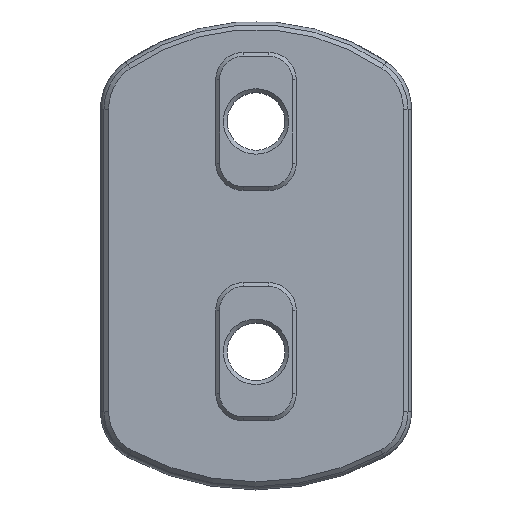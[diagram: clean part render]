
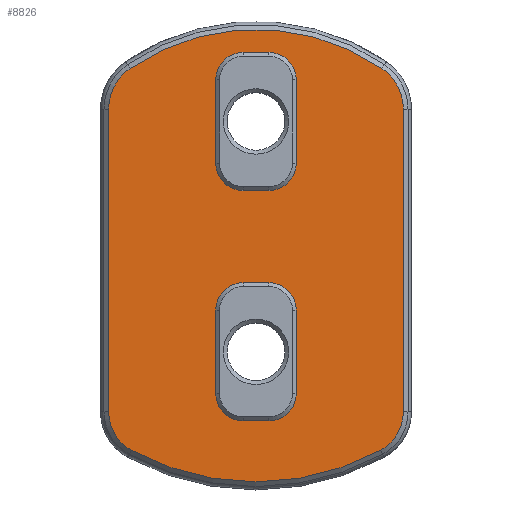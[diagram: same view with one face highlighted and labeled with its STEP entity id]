
A CAD part, top view. The second image highlights one B-rep face of the part: STEP entity #8826.
In plain terms, the highlighted planar face has unit normal (0, 0, 1).
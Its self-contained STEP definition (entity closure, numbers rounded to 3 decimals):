
#85=FACE_BOUND('',#2381,.T.);
#86=FACE_BOUND('',#2382,.T.);
#134=PLANE('',#9695);
#447=LINE('',#20648,#837);
#455=LINE('',#20966,#845);
#470=LINE('',#21016,#860);
#550=LINE('',#22989,#940);
#552=LINE('',#22998,#942);
#553=LINE('',#23002,#943);
#554=LINE('',#23005,#944);
#555=LINE('',#23007,#945);
#556=LINE('',#23009,#946);
#557=LINE('',#23013,#947);
#837=VECTOR('',#11187,10.);
#845=VECTOR('',#11223,10.);
#860=VECTOR('',#11274,10.);
#940=VECTOR('',#11726,10.);
#942=VECTOR('',#11738,10.);
#943=VECTOR('',#11741,10.);
#944=VECTOR('',#11744,10.);
#945=VECTOR('',#11745,10.);
#946=VECTOR('',#11746,10.);
#947=VECTOR('',#11749,10.);
#1774=FACE_OUTER_BOUND('',#2380,.T.);
#2380=EDGE_LOOP('',(#7814,#7815,#7816,#7817,#7818,#7819,#7820,#7821));
#2381=EDGE_LOOP('',(#7822,#7823,#7824,#7825,#7826,#7827,#7828,#7829));
#2382=EDGE_LOOP('',(#7830,#7831,#7832,#7833,#7834,#7835,#7836,#7837));
#2712=B_SPLINE_CURVE_WITH_KNOTS('',3,(#20640,#20641,#20642,#20643,#20644),
 .UNSPECIFIED.,.F.,.F.,(4,1,4),(0.,0.207,0.484),
 .UNSPECIFIED.);
#2804=B_SPLINE_CURVE_WITH_KNOTS('',3,(#22981,#22982,#22983,#22984,#22985),
 .UNSPECIFIED.,.F.,.F.,(4,1,4),(0.,0.207,0.484),
 .UNSPECIFIED.);
#3143=CIRCLE('',#9474,4.3);
#3150=CIRCLE('',#9484,2.38);
#3153=CIRCLE('',#9489,2.38);
#3160=CIRCLE('',#9503,2.38);
#3161=CIRCLE('',#9506,2.38);
#3261=CIRCLE('',#9689,22.602);
#3262=CIRCLE('',#9692,4.3);
#3263=CIRCLE('',#9694,19.302);
#3264=CIRCLE('',#9696,2.38);
#3265=CIRCLE('',#9697,2.38);
#3266=CIRCLE('',#9698,2.38);
#3267=CIRCLE('',#9699,2.38);
#3817=VERTEX_POINT('',#20637);
#3818=VERTEX_POINT('',#20639);
#3819=VERTEX_POINT('',#20647);
#3820=VERTEX_POINT('',#20651);
#3828=VERTEX_POINT('',#20953);
#3829=VERTEX_POINT('',#20954);
#3833=VERTEX_POINT('',#20964);
#3835=VERTEX_POINT('',#20970);
#3848=VERTEX_POINT('',#21009);
#3849=VERTEX_POINT('',#21011);
#3850=VERTEX_POINT('',#21015);
#3851=VERTEX_POINT('',#21019);
#3982=VERTEX_POINT('',#22956);
#3983=VERTEX_POINT('',#22979);
#3984=VERTEX_POINT('',#22987);
#3985=VERTEX_POINT('',#22991);
#3986=VERTEX_POINT('',#22997);
#3987=VERTEX_POINT('',#22999);
#3988=VERTEX_POINT('',#23001);
#3989=VERTEX_POINT('',#23003);
#3990=VERTEX_POINT('',#23006);
#3991=VERTEX_POINT('',#23008);
#3992=VERTEX_POINT('',#23010);
#3993=VERTEX_POINT('',#23012);
#4957=EDGE_CURVE('',#3818,#3817,#2712,.T.);
#4959=EDGE_CURVE('',#3819,#3818,#447,.T.);
#4961=EDGE_CURVE('',#3820,#3819,#3143,.T.);
#4981=EDGE_CURVE('',#3828,#3829,#3150,.T.);
#4987=EDGE_CURVE('',#3829,#3833,#455,.T.);
#4990=EDGE_CURVE('',#3835,#3833,#3153,.T.);
#5009=EDGE_CURVE('',#3849,#3848,#3160,.T.);
#5011=EDGE_CURVE('',#3850,#3849,#470,.T.);
#5013=EDGE_CURVE('',#3850,#3851,#3161,.T.);
#5269=EDGE_CURVE('',#3982,#3817,#3261,.T.);
#5271=EDGE_CURVE('',#3983,#3982,#2804,.T.);
#5273=EDGE_CURVE('',#3984,#3983,#550,.T.);
#5275=EDGE_CURVE('',#3985,#3984,#3262,.T.);
#5276=EDGE_CURVE('',#3985,#3820,#3263,.T.);
#5277=EDGE_CURVE('',#3986,#3848,#552,.T.);
#5278=EDGE_CURVE('',#3987,#3986,#3264,.T.);
#5279=EDGE_CURVE('',#3988,#3987,#553,.T.);
#5280=EDGE_CURVE('',#3988,#3989,#3265,.T.);
#5281=EDGE_CURVE('',#3851,#3989,#554,.T.);
#5282=EDGE_CURVE('',#3990,#3828,#555,.T.);
#5283=EDGE_CURVE('',#3991,#3835,#556,.T.);
#5284=EDGE_CURVE('',#3991,#3992,#3266,.T.);
#5285=EDGE_CURVE('',#3993,#3992,#557,.T.);
#5286=EDGE_CURVE('',#3990,#3993,#3267,.T.);
#7814=ORIENTED_EDGE('',*,*,#5276,.T.);
#7815=ORIENTED_EDGE('',*,*,#4961,.T.);
#7816=ORIENTED_EDGE('',*,*,#4959,.T.);
#7817=ORIENTED_EDGE('',*,*,#4957,.T.);
#7818=ORIENTED_EDGE('',*,*,#5269,.F.);
#7819=ORIENTED_EDGE('',*,*,#5271,.F.);
#7820=ORIENTED_EDGE('',*,*,#5273,.F.);
#7821=ORIENTED_EDGE('',*,*,#5275,.F.);
#7822=ORIENTED_EDGE('',*,*,#5277,.F.);
#7823=ORIENTED_EDGE('',*,*,#5278,.F.);
#7824=ORIENTED_EDGE('',*,*,#5279,.F.);
#7825=ORIENTED_EDGE('',*,*,#5280,.T.);
#7826=ORIENTED_EDGE('',*,*,#5281,.F.);
#7827=ORIENTED_EDGE('',*,*,#5013,.F.);
#7828=ORIENTED_EDGE('',*,*,#5011,.T.);
#7829=ORIENTED_EDGE('',*,*,#5009,.T.);
#7830=ORIENTED_EDGE('',*,*,#5282,.T.);
#7831=ORIENTED_EDGE('',*,*,#4981,.T.);
#7832=ORIENTED_EDGE('',*,*,#4987,.T.);
#7833=ORIENTED_EDGE('',*,*,#4990,.F.);
#7834=ORIENTED_EDGE('',*,*,#5283,.F.);
#7835=ORIENTED_EDGE('',*,*,#5284,.T.);
#7836=ORIENTED_EDGE('',*,*,#5285,.F.);
#7837=ORIENTED_EDGE('',*,*,#5286,.F.);
#8826=ADVANCED_FACE('',(#1774,#85,#86),#134,.F.);
#9474=AXIS2_PLACEMENT_3D('',#20652,#11191,#11192);
#9484=AXIS2_PLACEMENT_3D('',#20955,#11213,#11214);
#9489=AXIS2_PLACEMENT_3D('',#20972,#11229,#11230);
#9503=AXIS2_PLACEMENT_3D('',#21012,#11269,#11270);
#9506=AXIS2_PLACEMENT_3D('',#21020,#11278,#11279);
#9689=AXIS2_PLACEMENT_3D('',#22958,#11720,#11721);
#9692=AXIS2_PLACEMENT_3D('',#22993,#11730,#11731);
#9694=AXIS2_PLACEMENT_3D('',#22995,#11734,#11735);
#9695=AXIS2_PLACEMENT_3D('',#22996,#11736,#11737);
#9696=AXIS2_PLACEMENT_3D('',#23000,#11739,#11740);
#9697=AXIS2_PLACEMENT_3D('',#23004,#11742,#11743);
#9698=AXIS2_PLACEMENT_3D('',#23011,#11747,#11748);
#9699=AXIS2_PLACEMENT_3D('',#23014,#11750,#11751);
#11187=DIRECTION('',(0.,-1.,0.));
#11191=DIRECTION('center_axis',(0.,0.,1.));
#11192=DIRECTION('ref_axis',(-0.885,0.466,0.));
#11213=DIRECTION('center_axis',(0.,0.,
-1.));
#11214=DIRECTION('ref_axis',(-1.,0.,0.));
#11223=DIRECTION('',(0.,1.,0.));
#11229=DIRECTION('center_axis',(0.,0.,
1.));
#11230=DIRECTION('ref_axis',(0.,1.,0.));
#11269=DIRECTION('center_axis',(0.,0.,
-1.));
#11270=DIRECTION('ref_axis',(0.,1.,0.));
#11274=DIRECTION('',(0.,1.,0.));
#11278=DIRECTION('center_axis',(0.,0.,
1.));
#11279=DIRECTION('ref_axis',(-1.,0.,0.));
#11720=DIRECTION('center_axis',(0.,0.,-1.));
#11721=DIRECTION('ref_axis',(0.475,-0.88,0.));
#11726=DIRECTION('',(0.,-1.,0.));
#11730=DIRECTION('center_axis',(0.,0.,-1.));
#11731=DIRECTION('ref_axis',(0.885,0.466,0.));
#11734=DIRECTION('center_axis',(0.,0.,1.));
#11735=DIRECTION('ref_axis',(0.475,0.88,0.));
#11736=DIRECTION('center_axis',(0.,0.,-1.));
#11737=DIRECTION('ref_axis',(-1.,0.,0.));
#11738=DIRECTION('',(-1.,0.,0.));
#11739=DIRECTION('center_axis',(0.,0.,
1.));
#11740=DIRECTION('ref_axis',(0.,1.,0.));
#11741=DIRECTION('',(0.,1.,0.));
#11742=DIRECTION('center_axis',(0.,0.,
-1.));
#11743=DIRECTION('ref_axis',(1.,0.,0.));
#11744=DIRECTION('',(1.,0.,0.));
#11745=DIRECTION('',(-1.,0.,0.));
#11746=DIRECTION('',(-1.,0.,0.));
#11747=DIRECTION('center_axis',(0.,0.,
-1.));
#11748=DIRECTION('ref_axis',(0.,1.,0.));
#11749=DIRECTION('',(0.,1.,0.));
#11750=DIRECTION('center_axis',(0.,0.,
1.));
#11751=DIRECTION('ref_axis',(1.,0.,0.));
#20637=CARTESIAN_POINT('',(-10.819,-74.542,-2.8));
#20639=CARTESIAN_POINT('',(-12.8,-71.206,-2.8));
#20640=CARTESIAN_POINT('Ctrl Pts',(-12.8,-71.206,
-2.8));
#20641=CARTESIAN_POINT('Ctrl Pts',(-12.8,-71.789,
-2.8));
#20642=CARTESIAN_POINT('Ctrl Pts',(-12.483,-73.145,-2.8));
#20643=CARTESIAN_POINT('Ctrl Pts',(-11.502,-74.17,
-2.8));
#20644=CARTESIAN_POINT('Ctrl Pts',(-10.819,-74.542,
-2.8));
#20647=CARTESIAN_POINT('',(-12.8,-44.94,-2.8));
#20648=CARTESIAN_POINT('',(-12.8,-36.959,-2.8));
#20651=CARTESIAN_POINT('',(-10.936,-41.397,-2.8));
#20652=CARTESIAN_POINT('Origin',(-8.5,-44.94,-2.8));
#20953=CARTESIAN_POINT('',(-1.12,-72.,-2.8));
#20954=CARTESIAN_POINT('',(-3.5,-69.62,-2.8));
#20955=CARTESIAN_POINT('Origin',(-1.12,-69.62,-2.8));
#20964=CARTESIAN_POINT('',(-3.5,-62.38,-2.8));
#20966=CARTESIAN_POINT('',(-3.5,-69.62,-2.8));
#20970=CARTESIAN_POINT('',(-1.12,-60.,-2.8));
#20972=CARTESIAN_POINT('Origin',(-1.12,-62.38,-2.8));
#21009=CARTESIAN_POINT('',(-1.12,-40.,-2.8));
#21011=CARTESIAN_POINT('',(-3.5,-42.38,-2.8));
#21012=CARTESIAN_POINT('Origin',(-1.12,-42.38,-2.8));
#21015=CARTESIAN_POINT('',(-3.5,-49.62,-2.8));
#21016=CARTESIAN_POINT('',(-3.5,-69.62,-2.8));
#21019=CARTESIAN_POINT('',(-1.12,-52.,-2.8));
#21020=CARTESIAN_POINT('Origin',(-1.12,-49.62,-2.8));
#22956=CARTESIAN_POINT('',(10.819,-74.542,-2.8));
#22958=CARTESIAN_POINT('Origin',(0.,-54.698,
-2.8));
#22979=CARTESIAN_POINT('',(12.8,-71.206,-2.8));
#22981=CARTESIAN_POINT('Ctrl Pts',(12.8,-71.206,-2.8));
#22982=CARTESIAN_POINT('Ctrl Pts',(12.8,-71.789,-2.8));
#22983=CARTESIAN_POINT('Ctrl Pts',(12.483,-73.145,-2.8));
#22984=CARTESIAN_POINT('Ctrl Pts',(11.502,-74.17,-2.8));
#22985=CARTESIAN_POINT('Ctrl Pts',(10.819,-74.542,-2.8));
#22987=CARTESIAN_POINT('',(12.8,-44.94,-2.8));
#22989=CARTESIAN_POINT('',(12.8,-36.959,-2.8));
#22991=CARTESIAN_POINT('',(10.936,-41.397,-2.8));
#22993=CARTESIAN_POINT('Origin',(8.5,-44.94,-2.8));
#22995=CARTESIAN_POINT('Origin',(0.,-57.302,
-2.8));
#22996=CARTESIAN_POINT('Origin',(0.,-16.,-2.8));
#22997=CARTESIAN_POINT('',(1.12,-40.,-2.8));
#22998=CARTESIAN_POINT('',(1.12,-40.,-2.8));
#22999=CARTESIAN_POINT('',(3.5,-42.38,-2.8));
#23000=CARTESIAN_POINT('Origin',(1.12,-42.38,-2.8));
#23001=CARTESIAN_POINT('',(3.5,-49.62,-2.8));
#23002=CARTESIAN_POINT('',(3.5,-69.62,-2.8));
#23003=CARTESIAN_POINT('',(1.12,-52.,-2.8));
#23004=CARTESIAN_POINT('Origin',(1.12,-49.62,-2.8));
#23005=CARTESIAN_POINT('',(0.,-52.,-2.8));
#23006=CARTESIAN_POINT('',(1.12,-72.,-2.8));
#23007=CARTESIAN_POINT('',(0.56,-72.,-2.8));
#23008=CARTESIAN_POINT('',(1.12,-60.,-2.8));
#23009=CARTESIAN_POINT('',(0.,-60.,-2.8));
#23010=CARTESIAN_POINT('',(3.5,-62.38,-2.8));
#23011=CARTESIAN_POINT('Origin',(1.12,-62.38,-2.8));
#23012=CARTESIAN_POINT('',(3.5,-69.62,-2.8));
#23013=CARTESIAN_POINT('',(3.5,-69.62,-2.8));
#23014=CARTESIAN_POINT('Origin',(1.12,-69.62,-2.8));
